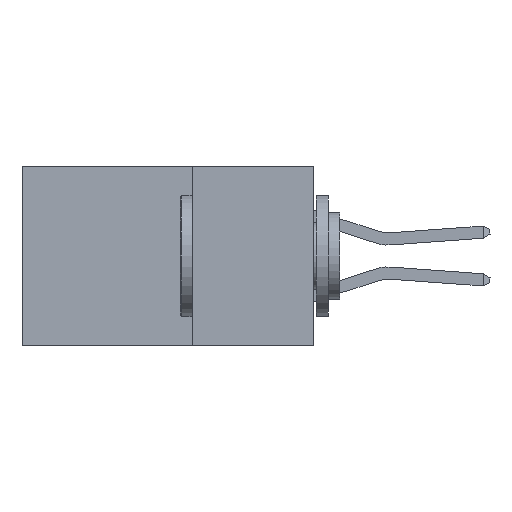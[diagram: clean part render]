
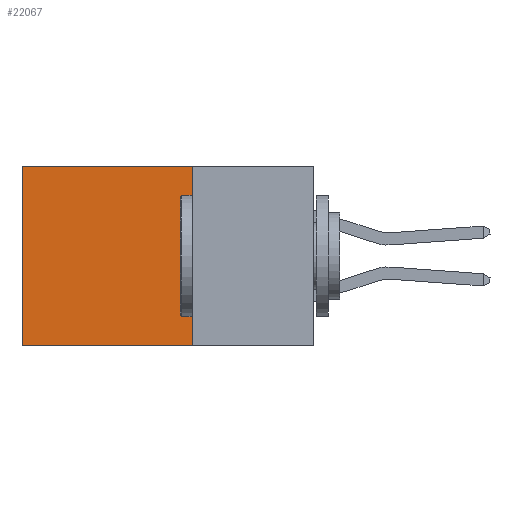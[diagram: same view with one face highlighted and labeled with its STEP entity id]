
A CAD part, left-side view. The second image highlights one B-rep face of the part: STEP entity #22067.
In plain terms, the highlighted planar face has unit normal (-1, 0, 0).
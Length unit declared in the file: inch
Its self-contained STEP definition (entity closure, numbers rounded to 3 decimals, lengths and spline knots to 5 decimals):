
#2577 = ORIENTED_EDGE ( 'NONE', *, *, #4518, .T. ) ;
#2857 = CARTESIAN_POINT ( 'NONE',  ( 0.2875, 0.6, -0.37 ) ) ;
#4048 = VECTOR ( 'NONE', #16319, 39.37008 ) ;
#4518 = EDGE_CURVE ( 'NONE', #29998, #31128, #14855, .T. ) ;
#4922 = LINE ( 'NONE', #21161, #4048 ) ;
#4931 = VECTOR ( 'NONE', #8138, 39.37008 ) ;
#8138 = DIRECTION ( 'NONE',  ( 0., 0., -1. ) ) ;
#8547 = ORIENTED_EDGE ( 'NONE', *, *, #32993, .T. ) ;
#8900 = CARTESIAN_POINT ( 'NONE',  ( 0.2875, 0.25, 0. ) ) ;
#11490 = DIRECTION ( 'NONE',  ( 1., 0., 0. ) ) ;
#11732 = CARTESIAN_POINT ( 'NONE',  ( 0.2875, 0.25, 0. ) ) ;
#11998 = DIRECTION ( 'NONE',  ( 0., 1., 0. ) ) ;
#12918 = VERTEX_POINT ( 'NONE', #8900 ) ;
#14254 = EDGE_CURVE ( 'NONE', #30345, #31128, #22746, .T. ) ;
#14793 = CARTESIAN_POINT ( 'NONE',  ( 0.2875, 0.25, 0. ) ) ;
#14855 = LINE ( 'NONE', #16767, #4931 ) ;
#15505 = EDGE_LOOP ( 'NONE', ( #2577, #26668, #16349, #8547 ) ) ;
#16319 = DIRECTION ( 'NONE',  ( 0., 1., 0. ) ) ;
#16349 = ORIENTED_EDGE ( 'NONE', *, *, #23509, .F. ) ;
#16767 = CARTESIAN_POINT ( 'NONE',  ( 0.2875, 0.6, 0. ) ) ;
#17231 = LINE ( 'NONE', #14793, #19010 ) ;
#18422 = AXIS2_PLACEMENT_3D ( 'NONE', #11732, #11490, #30678 ) ;
#18657 = CARTESIAN_POINT ( 'NONE',  ( 0.2875, 0.6, 0. ) ) ;
#19010 = VECTOR ( 'NONE', #31729, 39.37008 ) ;
#21161 = CARTESIAN_POINT ( 'NONE',  ( 0.2875, 0.25, 0. ) ) ;
#22067 = ADVANCED_FACE ( 'NONE', ( #32385 ), #27921, .F. ) ;
#22746 = LINE ( 'NONE', #28303, #27851 ) ;
#23509 = EDGE_CURVE ( 'NONE', #12918, #30345, #17231, .T. ) ;
#26668 = ORIENTED_EDGE ( 'NONE', *, *, #14254, .F. ) ;
#27851 = VECTOR ( 'NONE', #11998, 39.37008 ) ;
#27921 = PLANE ( 'NONE',  #18422 ) ;
#28073 = CARTESIAN_POINT ( 'NONE',  ( 0.2875, 0.25, -0.37 ) ) ;
#28303 = CARTESIAN_POINT ( 'NONE',  ( 0.2875, 0.25, -0.37 ) ) ;
#29998 = VERTEX_POINT ( 'NONE', #18657 ) ;
#30345 = VERTEX_POINT ( 'NONE', #28073 ) ;
#30678 = DIRECTION ( 'NONE',  ( 0., 0., -1. ) ) ;
#31128 = VERTEX_POINT ( 'NONE', #2857 ) ;
#31729 = DIRECTION ( 'NONE',  ( 0., 0., -1. ) ) ;
#32385 = FACE_OUTER_BOUND ( 'NONE', #15505, .T. ) ;
#32993 = EDGE_CURVE ( 'NONE', #12918, #29998, #4922, .T. ) ;
